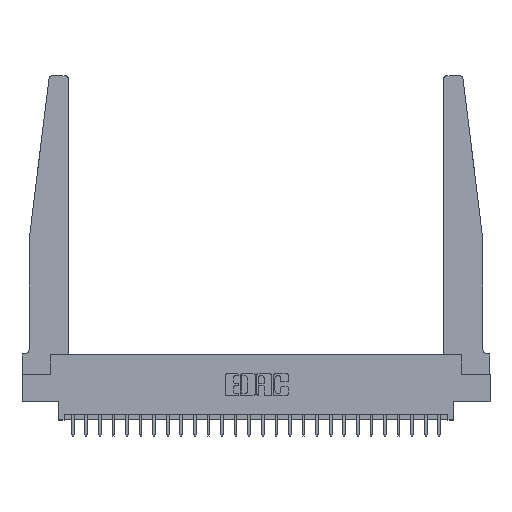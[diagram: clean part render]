
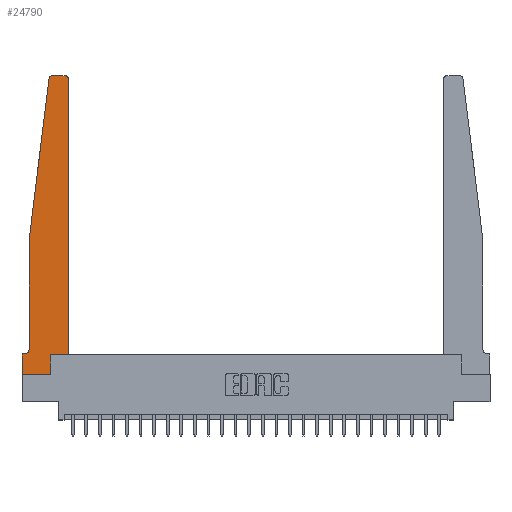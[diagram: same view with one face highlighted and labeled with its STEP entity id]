
A CAD part, top view. The second image highlights one B-rep face of the part: STEP entity #24790.
In plain terms, the highlighted planar face has unit normal (0, 0, 1).
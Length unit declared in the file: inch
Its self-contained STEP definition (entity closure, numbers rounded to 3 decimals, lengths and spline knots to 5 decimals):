
#5 = VECTOR ( 'NONE', #1540, 39.37008 ) ;
#432 = ORIENTED_EDGE ( 'NONE', *, *, #1101, .T. ) ;
#630 = DIRECTION ( 'NONE',  ( 0., 1., 0. ) ) ;
#1101 = EDGE_CURVE ( 'NONE', #8291, #19260, #12060, .T. ) ;
#1113 = CARTESIAN_POINT ( 'NONE',  ( 0.065, 1.25, 0.37 ) ) ;
#1344 = DIRECTION ( 'NONE',  ( 0., 0., 1. ) ) ;
#1401 = CARTESIAN_POINT ( 'NONE',  ( 0.425, 0.18, 0.37 ) ) ;
#1540 = DIRECTION ( 'NONE',  ( -1., 0., 0. ) ) ;
#1641 = ORIENTED_EDGE ( 'NONE', *, *, #14393, .T. ) ;
#1855 = AXIS2_PLACEMENT_3D ( 'NONE', #5861, #7679, #3786 ) ;
#2032 = ORIENTED_EDGE ( 'NONE', *, *, #19040, .T. ) ;
#2046 = EDGE_CURVE ( 'NONE', #14482, #3371, #24146, .T. ) ;
#2077 = VECTOR ( 'NONE', #20871, 39.37008 ) ;
#2508 = EDGE_CURVE ( 'NONE', #12593, #4628, #14694, .T. ) ;
#2811 = CARTESIAN_POINT ( 'NONE',  ( 0.2605, 0.18, 0.37 ) ) ;
#2896 = CARTESIAN_POINT ( 'NONE',  ( 0.395, 2.72, 0.37 ) ) ;
#2903 = AXIS2_PLACEMENT_3D ( 'NONE', #25304, #19091, #19463 ) ;
#3038 = CARTESIAN_POINT ( 'NONE',  ( 0.065, 1.25, 0.37 ) ) ;
#3168 = VERTEX_POINT ( 'NONE', #5155 ) ;
#3371 = VERTEX_POINT ( 'NONE', #3953 ) ;
#3415 = ORIENTED_EDGE ( 'NONE', *, *, #3430, .T. ) ;
#3430 = EDGE_CURVE ( 'NONE', #20089, #8291, #10032, .T. ) ;
#3539 = DIRECTION ( 'NONE',  ( 0., -1., 0. ) ) ;
#3786 = DIRECTION ( 'NONE',  ( 1., 0., 0. ) ) ;
#3953 = CARTESIAN_POINT ( 'NONE',  ( 0.425, 2.72, 0.37 ) ) ;
#4009 = FACE_OUTER_BOUND ( 'NONE', #5614, .T. ) ;
#4068 = CARTESIAN_POINT ( 'NONE',  ( 0., 0., 0.37 ) ) ;
#4264 = CARTESIAN_POINT ( 'NONE',  ( 0., 0.1875, 0.37 ) ) ;
#4628 = VERTEX_POINT ( 'NONE', #6557 ) ;
#5053 = VECTOR ( 'NONE', #17853, 39.37008 ) ;
#5155 = CARTESIAN_POINT ( 'NONE',  ( 0.015, 0.1875, 0.37 ) ) ;
#5284 = ORIENTED_EDGE ( 'NONE', *, *, #2508, .T. ) ;
#5508 = EDGE_CURVE ( 'NONE', #19260, #14482, #12775, .T. ) ;
#5579 = ORIENTED_EDGE ( 'NONE', *, *, #20792, .T. ) ;
#5614 = EDGE_LOOP ( 'NONE', ( #2032, #22237, #8917, #5284, #15458, #5579, #1641, #3415, #432, #11704, #5694, #10641 ) ) ;
#5694 = ORIENTED_EDGE ( 'NONE', *, *, #2046, .T. ) ;
#5861 = CARTESIAN_POINT ( 'NONE',  ( 0.27653, 2.72, 0.37 ) ) ;
#6361 = VERTEX_POINT ( 'NONE', #6667 ) ;
#6522 = EDGE_CURVE ( 'NONE', #3371, #12347, #17233, .T. ) ;
#6557 = CARTESIAN_POINT ( 'NONE',  ( 0.065, 0.2375, 0.37 ) ) ;
#6667 = CARTESIAN_POINT ( 'NONE',  ( 0.24675, 2.72367, 0.37 ) ) ;
#6672 = LINE ( 'NONE', #3038, #23215 ) ;
#7338 = VERTEX_POINT ( 'NONE', #20809 ) ;
#7589 = AXIS2_PLACEMENT_3D ( 'NONE', #4264, #15667, #23656 ) ;
#7679 = DIRECTION ( 'NONE',  ( 0., 0., 1. ) ) ;
#8163 = PLANE ( 'NONE',  #7589 ) ;
#8291 = VERTEX_POINT ( 'NONE', #9140 ) ;
#8917 = ORIENTED_EDGE ( 'NONE', *, *, #10039, .T. ) ;
#9140 = CARTESIAN_POINT ( 'NONE',  ( 0.2605, 0., 0.37 ) ) ;
#9653 = VECTOR ( 'NONE', #12387, 39.37008 ) ;
#10032 = LINE ( 'NONE', #4068, #15724 ) ;
#10039 = EDGE_CURVE ( 'NONE', #6361, #12593, #6672, .T. ) ;
#10553 = CARTESIAN_POINT ( 'NONE',  ( 0., 0., 0.37 ) ) ;
#10641 = ORIENTED_EDGE ( 'NONE', *, *, #6522, .T. ) ;
#11356 = CARTESIAN_POINT ( 'NONE',  ( 0.25, 2.75, 0.37 ) ) ;
#11590 = CARTESIAN_POINT ( 'NONE',  ( 0.395, 2.75, 0.37 ) ) ;
#11704 = ORIENTED_EDGE ( 'NONE', *, *, #5508, .T. ) ;
#11874 = CARTESIAN_POINT ( 'NONE',  ( 0.27653, 2.75, 0.37 ) ) ;
#12060 = LINE ( 'NONE', #21363, #18464 ) ;
#12347 = VERTEX_POINT ( 'NONE', #11590 ) ;
#12387 = DIRECTION ( 'NONE',  ( 1., 0., 0. ) ) ;
#12593 = VERTEX_POINT ( 'NONE', #18669 ) ;
#12716 = DIRECTION ( 'NONE',  ( 1., 0., 0. ) ) ;
#12775 = LINE ( 'NONE', #18062, #9653 ) ;
#13009 = CIRCLE ( 'NONE', #1855, 0.03 ) ;
#13873 = LINE ( 'NONE', #21728, #5053 ) ;
#14334 = CARTESIAN_POINT ( 'NONE',  ( 0.425, 0.18, 0.37 ) ) ;
#14393 = EDGE_CURVE ( 'NONE', #7338, #20089, #24999, .T. ) ;
#14482 = VERTEX_POINT ( 'NONE', #1401 ) ;
#14528 = EDGE_CURVE ( 'NONE', #19978, #6361, #13009, .T. ) ;
#14694 = LINE ( 'NONE', #1113, #2077 ) ;
#15458 = ORIENTED_EDGE ( 'NONE', *, *, #19035, .T. ) ;
#15513 = LINE ( 'NONE', #11356, #5 ) ;
#15667 = DIRECTION ( 'NONE',  ( 0., 0., 1. ) ) ;
#15724 = VECTOR ( 'NONE', #16704, 39.37008 ) ;
#16458 = DIRECTION ( 'NONE',  ( -0.122, -0.992, 0. ) ) ;
#16704 = DIRECTION ( 'NONE',  ( 1., 0., 0. ) ) ;
#17233 = CIRCLE ( 'NONE', #19287, 0.03 ) ;
#17853 = DIRECTION ( 'NONE',  ( -1., 0., 0. ) ) ;
#18062 = CARTESIAN_POINT ( 'NONE',  ( 0.425, 0.18, 0.37 ) ) ;
#18464 = VECTOR ( 'NONE', #24204, 39.37008 ) ;
#18669 = CARTESIAN_POINT ( 'NONE',  ( 0.065, 1.25, 0.37 ) ) ;
#19035 = EDGE_CURVE ( 'NONE', #4628, #3168, #23948, .T. ) ;
#19040 = EDGE_CURVE ( 'NONE', #12347, #19978, #15513, .T. ) ;
#19091 = DIRECTION ( 'NONE',  ( 0., 0., -1. ) ) ;
#19260 = VERTEX_POINT ( 'NONE', #2811 ) ;
#19287 = AXIS2_PLACEMENT_3D ( 'NONE', #2896, #1344, #12716 ) ;
#19463 = DIRECTION ( 'NONE',  ( -1., 0., 0. ) ) ;
#19978 = VERTEX_POINT ( 'NONE', #11874 ) ;
#20089 = VERTEX_POINT ( 'NONE', #10553 ) ;
#20792 = EDGE_CURVE ( 'NONE', #3168, #7338, #13873, .T. ) ;
#20809 = CARTESIAN_POINT ( 'NONE',  ( 0., 0.1875, 0.37 ) ) ;
#20871 = DIRECTION ( 'NONE',  ( 0., -1., 0. ) ) ;
#21226 = CARTESIAN_POINT ( 'NONE',  ( 0., 0., 0.37 ) ) ;
#21363 = CARTESIAN_POINT ( 'NONE',  ( 0.2605, 0.18, 0.37 ) ) ;
#21728 = CARTESIAN_POINT ( 'NONE',  ( 0.065, 0.1875, 0.37 ) ) ;
#22237 = ORIENTED_EDGE ( 'NONE', *, *, #14528, .T. ) ;
#23215 = VECTOR ( 'NONE', #16458, 39.37008 ) ;
#23656 = DIRECTION ( 'NONE',  ( 1., 0., 0. ) ) ;
#23922 = VECTOR ( 'NONE', #630, 39.37008 ) ;
#23948 = CIRCLE ( 'NONE', #2903, 0.05 ) ;
#24135 = VECTOR ( 'NONE', #3539, 39.37008 ) ;
#24146 = LINE ( 'NONE', #14334, #23922 ) ;
#24204 = DIRECTION ( 'NONE',  ( 0., 1., 0. ) ) ;
#24790 = ADVANCED_FACE ( 'NONE', ( #4009 ), #8163, .T. ) ;
#24999 = LINE ( 'NONE', #21226, #24135 ) ;
#25304 = CARTESIAN_POINT ( 'NONE',  ( 0.015, 0.2375, 0.37 ) ) ;
